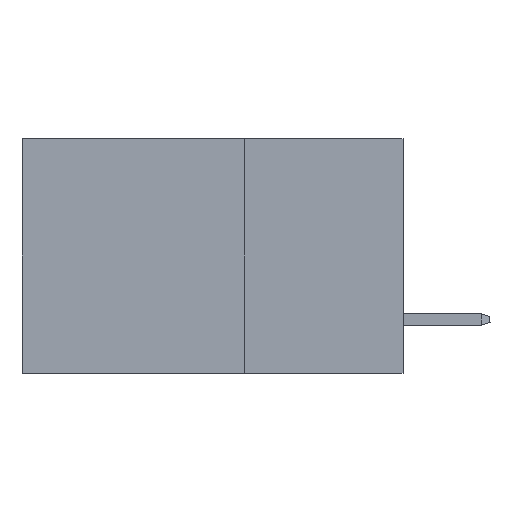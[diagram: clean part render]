
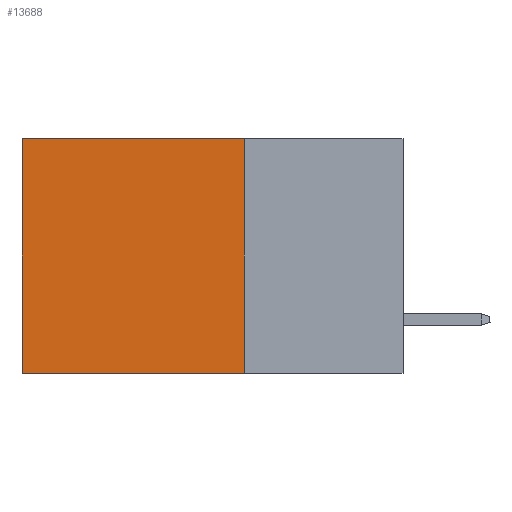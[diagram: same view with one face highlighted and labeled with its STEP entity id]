
A CAD part, left-side view. The second image highlights one B-rep face of the part: STEP entity #13688.
In plain terms, the highlighted planar face has unit normal (-1, 0, 0).
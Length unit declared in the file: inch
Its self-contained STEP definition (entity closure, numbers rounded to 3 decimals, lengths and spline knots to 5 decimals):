
#3637 = EDGE_CURVE ( 'NONE', #31337, #12855, #19238, .T. ) ;
#5871 = CARTESIAN_POINT ( 'NONE',  ( 0.2875, 0.25, -0.37 ) ) ;
#6318 = DIRECTION ( 'NONE',  ( 0., 0., -1. ) ) ;
#6620 = LINE ( 'NONE', #33674, #25110 ) ;
#6673 = VECTOR ( 'NONE', #6318, 39.37008 ) ;
#7477 = EDGE_CURVE ( 'NONE', #25583, #29702, #23092, .T. ) ;
#8874 = EDGE_CURVE ( 'NONE', #25583, #31337, #6620, .T. ) ;
#8944 = CARTESIAN_POINT ( 'NONE',  ( 0.2875, 0.6, 0. ) ) ;
#9864 = VECTOR ( 'NONE', #30818, 39.37008 ) ;
#9876 = EDGE_LOOP ( 'NONE', ( #31673, #10986, #19694, #27454 ) ) ;
#10590 = FACE_OUTER_BOUND ( 'NONE', #9876, .T. ) ;
#10773 = PLANE ( 'NONE',  #21921 ) ;
#10986 = ORIENTED_EDGE ( 'NONE', *, *, #3637, .F. ) ;
#11751 = LINE ( 'NONE', #8944, #6673 ) ;
#12855 = VERTEX_POINT ( 'NONE', #32453 ) ;
#13250 = VECTOR ( 'NONE', #16595, 39.37008 ) ;
#13688 = ADVANCED_FACE ( 'NONE', ( #10590 ), #10773, .F. ) ;
#14127 = CARTESIAN_POINT ( 'NONE',  ( 0.2875, 0.25, 0. ) ) ;
#16595 = DIRECTION ( 'NONE',  ( 0., 1., 0. ) ) ;
#18507 = CARTESIAN_POINT ( 'NONE',  ( 0.2875, 0.25, 0. ) ) ;
#19238 = LINE ( 'NONE', #5871, #13250 ) ;
#19694 = ORIENTED_EDGE ( 'NONE', *, *, #8874, .F. ) ;
#20348 = CARTESIAN_POINT ( 'NONE',  ( 0.2875, 0.6, 0. ) ) ;
#20475 = CARTESIAN_POINT ( 'NONE',  ( 0.2875, 0.25, -0.37 ) ) ;
#21319 = DIRECTION ( 'NONE',  ( 0., 0., -1. ) ) ;
#21921 = AXIS2_PLACEMENT_3D ( 'NONE', #18507, #29237, #21319 ) ;
#22629 = DIRECTION ( 'NONE',  ( 0., 0., -1. ) ) ;
#22739 = CARTESIAN_POINT ( 'NONE',  ( 0.2875, 0.25, 0. ) ) ;
#22846 = EDGE_CURVE ( 'NONE', #29702, #12855, #11751, .T. ) ;
#23092 = LINE ( 'NONE', #22739, #9864 ) ;
#25110 = VECTOR ( 'NONE', #22629, 39.37008 ) ;
#25583 = VERTEX_POINT ( 'NONE', #14127 ) ;
#27454 = ORIENTED_EDGE ( 'NONE', *, *, #7477, .T. ) ;
#29237 = DIRECTION ( 'NONE',  ( 1., 0., 0. ) ) ;
#29702 = VERTEX_POINT ( 'NONE', #20348 ) ;
#30818 = DIRECTION ( 'NONE',  ( 0., 1., 0. ) ) ;
#31337 = VERTEX_POINT ( 'NONE', #20475 ) ;
#31673 = ORIENTED_EDGE ( 'NONE', *, *, #22846, .T. ) ;
#32453 = CARTESIAN_POINT ( 'NONE',  ( 0.2875, 0.6, -0.37 ) ) ;
#33674 = CARTESIAN_POINT ( 'NONE',  ( 0.2875, 0.25, 0. ) ) ;
